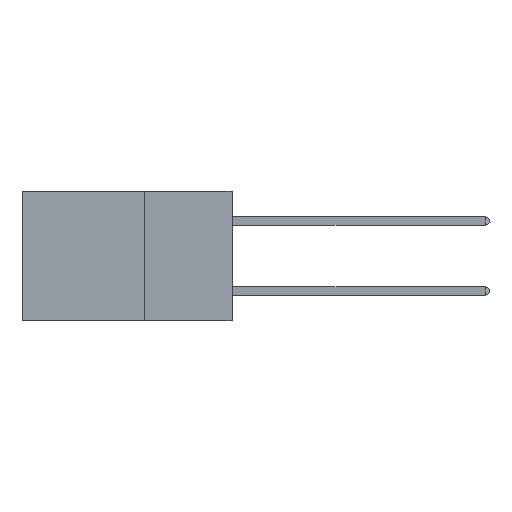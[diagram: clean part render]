
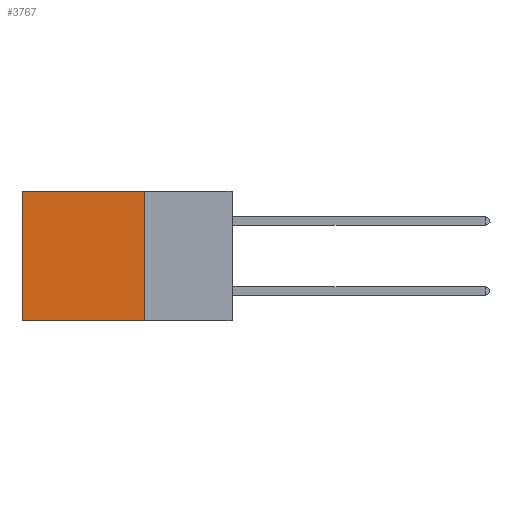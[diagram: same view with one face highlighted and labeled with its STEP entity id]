
A CAD part, left-side view. The second image highlights one B-rep face of the part: STEP entity #3767.
In plain terms, the highlighted planar face has unit normal (-1, 0, 0).
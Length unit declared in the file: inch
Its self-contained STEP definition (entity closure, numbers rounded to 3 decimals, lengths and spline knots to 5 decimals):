
#73 = VECTOR ( 'NONE', #3432, 39.37008 ) ;
#360 = ORIENTED_EDGE ( 'NONE', *, *, #5622, .T. ) ;
#1084 = VECTOR ( 'NONE', #8126, 39.37008 ) ;
#1623 = EDGE_LOOP ( 'NONE', ( #1996, #6963, #6415, #360 ) ) ;
#1799 = PLANE ( 'NONE',  #16099 ) ;
#1996 = ORIENTED_EDGE ( 'NONE', *, *, #7162, .T. ) ;
#2861 = CARTESIAN_POINT ( 'NONE',  ( 0.2875, 0.6, 0. ) ) ;
#3432 = DIRECTION ( 'NONE',  ( 0., 1., 0. ) ) ;
#3573 = EDGE_CURVE ( 'NONE', #16645, #9377, #9427, .T. ) ;
#3767 = ADVANCED_FACE ( 'NONE', ( #7603 ), #1799, .F. ) ;
#3806 = CARTESIAN_POINT ( 'NONE',  ( 0.2875, 0.25, 0. ) ) ;
#3882 = DIRECTION ( 'NONE',  ( 0., 1., 0. ) ) ;
#4316 = VERTEX_POINT ( 'NONE', #2861 ) ;
#4326 = VECTOR ( 'NONE', #3882, 39.37008 ) ;
#4851 = VECTOR ( 'NONE', #10601, 39.37008 ) ;
#5622 = EDGE_CURVE ( 'NONE', #14489, #4316, #9155, .T. ) ;
#6415 = ORIENTED_EDGE ( 'NONE', *, *, #11733, .F. ) ;
#6963 = ORIENTED_EDGE ( 'NONE', *, *, #3573, .F. ) ;
#7162 = EDGE_CURVE ( 'NONE', #4316, #9377, #10585, .T. ) ;
#7450 = CARTESIAN_POINT ( 'NONE',  ( 0.2875, 0.25, 0. ) ) ;
#7603 = FACE_OUTER_BOUND ( 'NONE', #1623, .T. ) ;
#8126 = DIRECTION ( 'NONE',  ( 0., 0., -1. ) ) ;
#8458 = DIRECTION ( 'NONE',  ( 0., 0., -1. ) ) ;
#9155 = LINE ( 'NONE', #7450, #73 ) ;
#9377 = VERTEX_POINT ( 'NONE', #16033 ) ;
#9427 = LINE ( 'NONE', #16934, #4326 ) ;
#10585 = LINE ( 'NONE', #16039, #1084 ) ;
#10601 = DIRECTION ( 'NONE',  ( 0., 0., -1. ) ) ;
#11082 = DIRECTION ( 'NONE',  ( 1., 0., 0. ) ) ;
#11733 = EDGE_CURVE ( 'NONE', #14489, #16645, #15557, .T. ) ;
#13798 = CARTESIAN_POINT ( 'NONE',  ( 0.2875, 0.25, -0.37 ) ) ;
#14315 = CARTESIAN_POINT ( 'NONE',  ( 0.2875, 0.25, 0. ) ) ;
#14489 = VERTEX_POINT ( 'NONE', #14315 ) ;
#15557 = LINE ( 'NONE', #3806, #4851 ) ;
#16033 = CARTESIAN_POINT ( 'NONE',  ( 0.2875, 0.6, -0.37 ) ) ;
#16039 = CARTESIAN_POINT ( 'NONE',  ( 0.2875, 0.6, 0. ) ) ;
#16099 = AXIS2_PLACEMENT_3D ( 'NONE', #16363, #11082, #8458 ) ;
#16363 = CARTESIAN_POINT ( 'NONE',  ( 0.2875, 0.25, 0. ) ) ;
#16645 = VERTEX_POINT ( 'NONE', #13798 ) ;
#16934 = CARTESIAN_POINT ( 'NONE',  ( 0.2875, 0.25, -0.37 ) ) ;
